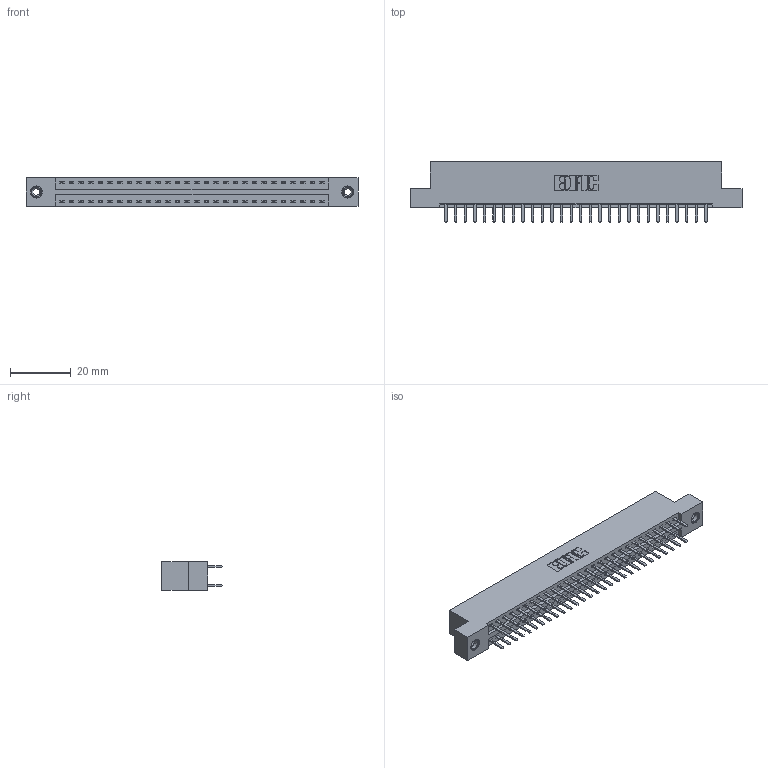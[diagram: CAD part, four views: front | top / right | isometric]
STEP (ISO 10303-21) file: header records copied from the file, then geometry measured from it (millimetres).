
FILE_DESCRIPTION (( 'STEP AP203' ), '1' );
FILE_NAME ('396-056-520-208.STEP', '2018-09-08T09:04:34', ( '' ), ( '' ), 'SwSTEP 2.0', 'SolidWorks 2016', '' );
FILE_SCHEMA (( 'CONFIG_CONTROL_DESIGN' ));
Length unit declared in the file: inch
Products named in the file (4): 345-250-001_345-250-003-102; 396-056-520-208; 346 Part_Flush Mounting Lugs - 0.156 Dia-TI; 345-292-001_345-293-120
Assembly tree (59 placements, depth 2):
  396-056-520-208
    346 Part_Flush Mounting Lugs - 0.156 Dia-TI
    345-292-001_345-293-120  x56
    345-250-001_345-250-003-102  x2
Bounding box: 109.47 x 20.02 x 9.4 mm (x, y, z)
Volume: 10535.2 mm3; surface area: 14223.6 mm2
Topology: 59 solids, 59 shells, 3318 faces, 9593 edges, 6238 vertices
Faces by surface type: plane 2180, cylinder 1122, cone 12, torus 4
Entity records: 21458 total; most frequent: CARTESIAN_POINT 3551, ORIENTED_EDGE 3466, DIRECTION 3195, EDGE_CURVE 1733, VECTOR 1465, LINE 1465, VERTEX_POINT 1148, AXIS2_PLACEMENT_3D 865
